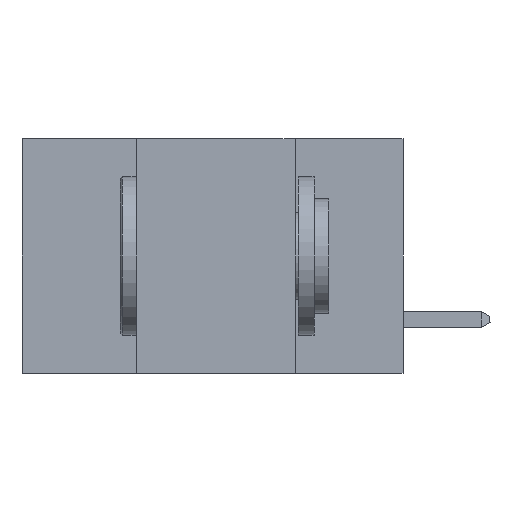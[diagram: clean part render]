
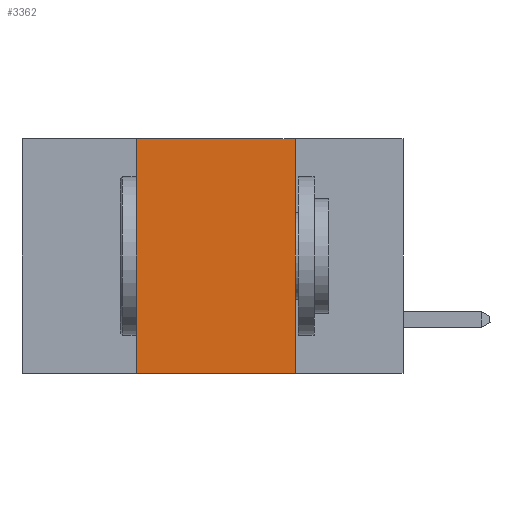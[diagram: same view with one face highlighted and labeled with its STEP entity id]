
A CAD part, left-side view. The second image highlights one B-rep face of the part: STEP entity #3362.
In plain terms, the highlighted planar face has unit normal (-1, 0, 0).
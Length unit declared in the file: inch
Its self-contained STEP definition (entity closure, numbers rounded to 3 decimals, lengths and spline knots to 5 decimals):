
#801 = CARTESIAN_POINT ( 'NONE',  ( 0., 0.17, 0. ) ) ;
#2725 = CARTESIAN_POINT ( 'NONE',  ( 0., 0.42, -0.37 ) ) ;
#3362 = ADVANCED_FACE ( 'NONE', ( #23727 ), #22803, .F. ) ;
#4323 = CARTESIAN_POINT ( 'NONE',  ( 0., 0.6, -0.37 ) ) ;
#4585 = CARTESIAN_POINT ( 'NONE',  ( 0., 0.6, 0. ) ) ;
#5279 = EDGE_LOOP ( 'NONE', ( #27668, #20281, #13203, #6166 ) ) ;
#5712 = CARTESIAN_POINT ( 'NONE',  ( 0., 0.42, 0. ) ) ;
#6166 = ORIENTED_EDGE ( 'NONE', *, *, #6618, .T. ) ;
#6618 = EDGE_CURVE ( 'NONE', #11407, #14779, #12157, .T. ) ;
#6767 = EDGE_CURVE ( 'NONE', #28508, #14779, #19945, .T. ) ;
#8908 = VECTOR ( 'NONE', #26167, 39.37008 ) ;
#8958 = VECTOR ( 'NONE', #13876, 39.37008 ) ;
#9343 = DIRECTION ( 'NONE',  ( 0., 0., -1. ) ) ;
#9449 = CARTESIAN_POINT ( 'NONE',  ( 0., 0.42, 0. ) ) ;
#11407 = VERTEX_POINT ( 'NONE', #2725 ) ;
#12157 = LINE ( 'NONE', #4323, #21717 ) ;
#13203 = ORIENTED_EDGE ( 'NONE', *, *, #24322, .F. ) ;
#13723 = CARTESIAN_POINT ( 'NONE',  ( 0., 0.6, 0. ) ) ;
#13817 = DIRECTION ( 'NONE',  ( 1., 0., 0. ) ) ;
#13876 = DIRECTION ( 'NONE',  ( 0., -1., 0. ) ) ;
#14779 = VERTEX_POINT ( 'NONE', #22163 ) ;
#17391 = VERTEX_POINT ( 'NONE', #9449 ) ;
#17731 = CARTESIAN_POINT ( 'NONE',  ( 0., 0.17, 0. ) ) ;
#18843 = VECTOR ( 'NONE', #26652, 39.37008 ) ;
#19931 = LINE ( 'NONE', #4585, #8958 ) ;
#19945 = LINE ( 'NONE', #17731, #18843 ) ;
#20281 = ORIENTED_EDGE ( 'NONE', *, *, #23799, .F. ) ;
#21717 = VECTOR ( 'NONE', #22418, 39.37008 ) ;
#22163 = CARTESIAN_POINT ( 'NONE',  ( 0., 0.17, -0.37 ) ) ;
#22182 = AXIS2_PLACEMENT_3D ( 'NONE', #13723, #13817, #9343 ) ;
#22418 = DIRECTION ( 'NONE',  ( 0., -1., 0. ) ) ;
#22803 = PLANE ( 'NONE',  #22182 ) ;
#23727 = FACE_OUTER_BOUND ( 'NONE', #5279, .T. ) ;
#23799 = EDGE_CURVE ( 'NONE', #17391, #28508, #19931, .T. ) ;
#24322 = EDGE_CURVE ( 'NONE', #11407, #17391, #27667, .T. ) ;
#26167 = DIRECTION ( 'NONE',  ( 0., 0., 1. ) ) ;
#26652 = DIRECTION ( 'NONE',  ( 0., 0., -1. ) ) ;
#27667 = LINE ( 'NONE', #5712, #8908 ) ;
#27668 = ORIENTED_EDGE ( 'NONE', *, *, #6767, .F. ) ;
#28508 = VERTEX_POINT ( 'NONE', #801 ) ;
